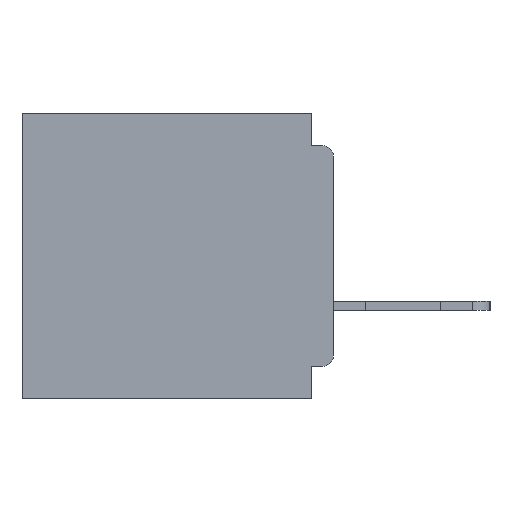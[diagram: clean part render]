
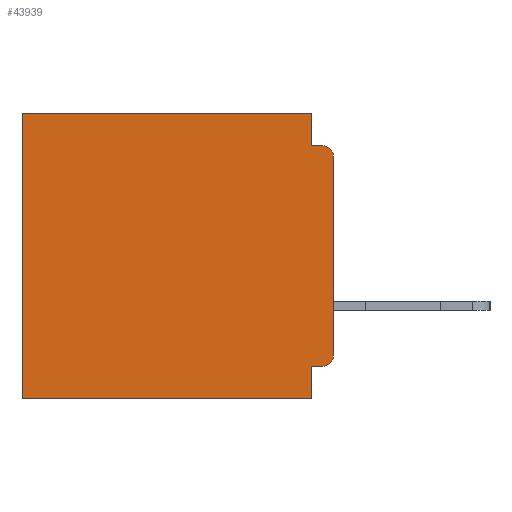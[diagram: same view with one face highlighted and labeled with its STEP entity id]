
A CAD part, left-side view. The second image highlights one B-rep face of the part: STEP entity #43939.
In plain terms, the highlighted planar face has unit normal (-1, 0, 0).
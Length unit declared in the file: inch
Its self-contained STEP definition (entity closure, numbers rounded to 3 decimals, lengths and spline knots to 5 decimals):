
#1786 = VECTOR ( 'NONE', #20121, 39.37008 ) ;
#2068 = LINE ( 'NONE', #26298, #18967 ) ;
#2081 = VERTEX_POINT ( 'NONE', #41404 ) ;
#2239 = EDGE_CURVE ( 'NONE', #2081, #4930, #28794, .T. ) ;
#2615 = CARTESIAN_POINT ( 'NONE',  ( 0.3, 0.031, 0. ) ) ;
#2840 = DIRECTION ( 'NONE',  ( 0., 0., -1. ) ) ;
#3900 = VECTOR ( 'NONE', #41346, 39.37008 ) ;
#4152 = EDGE_CURVE ( 'NONE', #23660, #4930, #2068, .T. ) ;
#4327 = CARTESIAN_POINT ( 'NONE',  ( 0.3, 0., -0.34 ) ) ;
#4930 = VERTEX_POINT ( 'NONE', #27390 ) ;
#5642 = PLANE ( 'NONE',  #22877 ) ;
#5977 = ORIENTED_EDGE ( 'NONE', *, *, #16888, .F. ) ;
#6323 = CIRCLE ( 'NONE', #24837, 0.015 ) ;
#6513 = CARTESIAN_POINT ( 'NONE',  ( 0.3, 0., 0. ) ) ;
#7213 = LINE ( 'NONE', #12416, #24172 ) ;
#7217 = VECTOR ( 'NONE', #42909, 39.37008 ) ;
#7802 = EDGE_CURVE ( 'NONE', #24126, #2081, #21888, .T. ) ;
#8491 = ORIENTED_EDGE ( 'NONE', *, *, #25187, .F. ) ;
#10268 = VERTEX_POINT ( 'NONE', #36204 ) ;
#11726 = ORIENTED_EDGE ( 'NONE', *, *, #42027, .T. ) ;
#12416 = CARTESIAN_POINT ( 'NONE',  ( 0.3, 0., -0.4 ) ) ;
#13125 = EDGE_CURVE ( 'NONE', #21354, #14811, #24324, .T. ) ;
#14692 = DIRECTION ( 'NONE',  ( 0., -1., 0. ) ) ;
#14811 = VERTEX_POINT ( 'NONE', #28487 ) ;
#15290 = VECTOR ( 'NONE', #43651, 39.37008 ) ;
#15473 = EDGE_LOOP ( 'NONE', ( #5977, #37520, #8491, #26973, #11726, #37700, #21892, #38575, #36444, #26087 ) ) ;
#15563 = EDGE_CURVE ( 'NONE', #10268, #17745, #41296, .T. ) ;
#15779 = DIRECTION ( 'NONE',  ( 0., 0., -1. ) ) ;
#15851 = DIRECTION ( 'NONE',  ( 0., 0., -1. ) ) ;
#16204 = LINE ( 'NONE', #22565, #7217 ) ;
#16888 = EDGE_CURVE ( 'NONE', #31698, #17745, #7213, .T. ) ;
#17538 = LINE ( 'NONE', #6513, #25475 ) ;
#17728 = CARTESIAN_POINT ( 'NONE',  ( 0.3, 0.015, -0.06 ) ) ;
#17745 = VERTEX_POINT ( 'NONE', #4327 ) ;
#18967 = VECTOR ( 'NONE', #26689, 39.37008 ) ;
#19501 = FACE_OUTER_BOUND ( 'NONE', #15473, .T. ) ;
#19644 = VECTOR ( 'NONE', #14692, 39.37008 ) ;
#20121 = DIRECTION ( 'NONE',  ( 0., 1., 0. ) ) ;
#21108 = DIRECTION ( 'NONE',  ( 0., 0., -1. ) ) ;
#21354 = VERTEX_POINT ( 'NONE', #2615 ) ;
#21888 = LINE ( 'NONE', #41545, #3900 ) ;
#21892 = ORIENTED_EDGE ( 'NONE', *, *, #2239, .F. ) ;
#22043 = AXIS2_PLACEMENT_3D ( 'NONE', #43453, #23093, #2840 ) ;
#22565 = CARTESIAN_POINT ( 'NONE',  ( 0.3, 0., -0.355 ) ) ;
#22877 = AXIS2_PLACEMENT_3D ( 'NONE', #42883, #36190, #15851 ) ;
#23093 = DIRECTION ( 'NONE',  ( -1., 0., 0. ) ) ;
#23660 = VERTEX_POINT ( 'NONE', #40505 ) ;
#24126 = VERTEX_POINT ( 'NONE', #26064 ) ;
#24172 = VECTOR ( 'NONE', #15779, 39.37008 ) ;
#24324 = LINE ( 'NONE', #29981, #15290 ) ;
#24837 = AXIS2_PLACEMENT_3D ( 'NONE', #17728, #41471, #21108 ) ;
#24923 = CARTESIAN_POINT ( 'NONE',  ( 0.3, 0., -0.045 ) ) ;
#25187 = EDGE_CURVE ( 'NONE', #14811, #31058, #37738, .T. ) ;
#25475 = VECTOR ( 'NONE', #40476, 39.37008 ) ;
#25594 = CARTESIAN_POINT ( 'NONE',  ( 0.3, 0., -0.06 ) ) ;
#26064 = CARTESIAN_POINT ( 'NONE',  ( 0.3, 0.031, -0.355 ) ) ;
#26087 = ORIENTED_EDGE ( 'NONE', *, *, #15563, .T. ) ;
#26221 = EDGE_CURVE ( 'NONE', #31698, #31058, #6323, .T. ) ;
#26298 = CARTESIAN_POINT ( 'NONE',  ( 0.3, 0.437, -0.4 ) ) ;
#26689 = DIRECTION ( 'NONE',  ( 0., 0., -1. ) ) ;
#26973 = ORIENTED_EDGE ( 'NONE', *, *, #13125, .F. ) ;
#27390 = CARTESIAN_POINT ( 'NONE',  ( 0.3, 0.437, -0.4 ) ) ;
#28487 = CARTESIAN_POINT ( 'NONE',  ( 0.3, 0.031, -0.045 ) ) ;
#28794 = LINE ( 'NONE', #29950, #1786 ) ;
#29950 = CARTESIAN_POINT ( 'NONE',  ( 0.3, 0., -0.4 ) ) ;
#29981 = CARTESIAN_POINT ( 'NONE',  ( 0.3, 0.031, 0. ) ) ;
#31058 = VERTEX_POINT ( 'NONE', #32350 ) ;
#31698 = VERTEX_POINT ( 'NONE', #25594 ) ;
#32350 = CARTESIAN_POINT ( 'NONE',  ( 0.3, 0.015, -0.045 ) ) ;
#32369 = EDGE_CURVE ( 'NONE', #10268, #24126, #16204, .T. ) ;
#36190 = DIRECTION ( 'NONE',  ( 1., 0., 0. ) ) ;
#36204 = CARTESIAN_POINT ( 'NONE',  ( 0.3, 0.015, -0.355 ) ) ;
#36444 = ORIENTED_EDGE ( 'NONE', *, *, #32369, .F. ) ;
#37520 = ORIENTED_EDGE ( 'NONE', *, *, #26221, .T. ) ;
#37700 = ORIENTED_EDGE ( 'NONE', *, *, #4152, .T. ) ;
#37738 = LINE ( 'NONE', #24923, #19644 ) ;
#38575 = ORIENTED_EDGE ( 'NONE', *, *, #7802, .F. ) ;
#40476 = DIRECTION ( 'NONE',  ( 0., 1., 0. ) ) ;
#40505 = CARTESIAN_POINT ( 'NONE',  ( 0.3, 0.437, 0. ) ) ;
#41296 = CIRCLE ( 'NONE', #22043, 0.015 ) ;
#41346 = DIRECTION ( 'NONE',  ( 0., 0., -1. ) ) ;
#41404 = CARTESIAN_POINT ( 'NONE',  ( 0.3, 0.031, -0.4 ) ) ;
#41471 = DIRECTION ( 'NONE',  ( -1., 0., 0. ) ) ;
#41545 = CARTESIAN_POINT ( 'NONE',  ( 0.3, 0.031, -0.4 ) ) ;
#42027 = EDGE_CURVE ( 'NONE', #21354, #23660, #17538, .T. ) ;
#42883 = CARTESIAN_POINT ( 'NONE',  ( 0.3, 0., -0.4 ) ) ;
#42909 = DIRECTION ( 'NONE',  ( 0., 1., 0. ) ) ;
#43453 = CARTESIAN_POINT ( 'NONE',  ( 0.3, 0.015, -0.34 ) ) ;
#43651 = DIRECTION ( 'NONE',  ( 0., 0., -1. ) ) ;
#43939 = ADVANCED_FACE ( 'NONE', ( #19501 ), #5642, .F. ) ;
